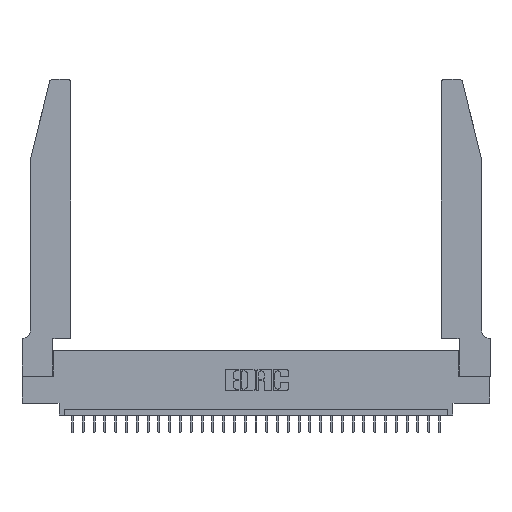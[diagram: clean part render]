
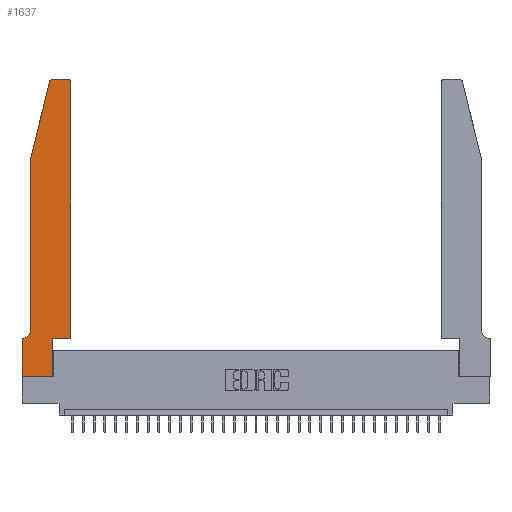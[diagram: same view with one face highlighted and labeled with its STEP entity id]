
A CAD part, top view. The second image highlights one B-rep face of the part: STEP entity #1637.
In plain terms, the highlighted planar face has unit normal (0, 0, 1).
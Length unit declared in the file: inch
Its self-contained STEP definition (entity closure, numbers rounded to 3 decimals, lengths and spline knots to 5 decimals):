
#861 = EDGE_CURVE ( 'NONE', #22324, #21856, #28466, .T. ) ;
#1229 = ORIENTED_EDGE ( 'NONE', *, *, #14745, .T. ) ;
#1288 = LINE ( 'NONE', #3930, #5575 ) ;
#1637 = ADVANCED_FACE ( 'NONE', ( #19854 ), #12151, .T. ) ;
#2127 = CARTESIAN_POINT ( 'NONE',  ( 0.0755, 2., 0.37 ) ) ;
#2329 = CARTESIAN_POINT ( 'NONE',  ( 0., 0.35, 0.37 ) ) ;
#2331 = CARTESIAN_POINT ( 'NONE',  ( 0.284, 2.72, 0.37 ) ) ;
#2631 = VERTEX_POINT ( 'NONE', #12043 ) ;
#2893 = VECTOR ( 'NONE', #9848, 39.37008 ) ;
#2916 = CARTESIAN_POINT ( 'NONE',  ( 0.2865, 0., 0.37 ) ) ;
#3930 = CARTESIAN_POINT ( 'NONE',  ( 0.0755, 0.35, 0.37 ) ) ;
#5282 = ORIENTED_EDGE ( 'NONE', *, *, #9246, .T. ) ;
#5521 = CARTESIAN_POINT ( 'NONE',  ( 0.0755, 2., 0.37 ) ) ;
#5575 = VECTOR ( 'NONE', #19083, 39.37008 ) ;
#5857 = EDGE_CURVE ( 'NONE', #2631, #22324, #8722, .T. ) ;
#5982 = DIRECTION ( 'NONE',  ( 0., 0., 1. ) ) ;
#6143 = CIRCLE ( 'NONE', #31142, 0.03 ) ;
#6165 = LINE ( 'NONE', #23189, #31897 ) ;
#6325 = VERTEX_POINT ( 'NONE', #20496 ) ;
#6509 = EDGE_CURVE ( 'NONE', #28198, #23085, #9923, .T. ) ;
#6625 = DIRECTION ( 'NONE',  ( 0., 0., -1. ) ) ;
#6813 = VERTEX_POINT ( 'NONE', #10339 ) ;
#6814 = EDGE_CURVE ( 'NONE', #6325, #8275, #25133, .T. ) ;
#7172 = CARTESIAN_POINT ( 'NONE',  ( 0.2865, 0.35, 0.37 ) ) ;
#7774 = AXIS2_PLACEMENT_3D ( 'NONE', #2329, #31929, #21804 ) ;
#8275 = VERTEX_POINT ( 'NONE', #2916 ) ;
#8722 = CIRCLE ( 'NONE', #31695, 0.03 ) ;
#9246 = EDGE_CURVE ( 'NONE', #29948, #19642, #29236, .T. ) ;
#9638 = LINE ( 'NONE', #16911, #32216 ) ;
#9848 = DIRECTION ( 'NONE',  ( 1., 0., 0. ) ) ;
#9882 = DIRECTION ( 'NONE',  ( 1., 0., 0. ) ) ;
#9923 = LINE ( 'NONE', #29613, #12692 ) ;
#9952 = DIRECTION ( 'NONE',  ( 1., 0., 0. ) ) ;
#9966 = CARTESIAN_POINT ( 'NONE',  ( 0., 0.35, 0.37 ) ) ;
#10187 = ORIENTED_EDGE ( 'NONE', *, *, #26667, .T. ) ;
#10339 = CARTESIAN_POINT ( 'NONE',  ( 0.0755, 0.42, 0.37 ) ) ;
#12043 = CARTESIAN_POINT ( 'NONE',  ( 0.4505, 2.72, 0.37 ) ) ;
#12145 = DIRECTION ( 'NONE',  ( 0., 1., 0. ) ) ;
#12151 = PLANE ( 'NONE',  #7774 ) ;
#12428 = ORIENTED_EDGE ( 'NONE', *, *, #6509, .T. ) ;
#12692 = VECTOR ( 'NONE', #9882, 39.37008 ) ;
#13392 = ORIENTED_EDGE ( 'NONE', *, *, #27468, .T. ) ;
#13490 = DIRECTION ( 'NONE',  ( 0., 1., 0. ) ) ;
#14745 = EDGE_CURVE ( 'NONE', #23166, #6325, #21315, .T. ) ;
#15244 = VECTOR ( 'NONE', #21880, 39.37008 ) ;
#16212 = CARTESIAN_POINT ( 'NONE',  ( 0.4205, 2.75, 0.37 ) ) ;
#16665 = CARTESIAN_POINT ( 'NONE',  ( 0.2605, 2.75, 0.37 ) ) ;
#16911 = CARTESIAN_POINT ( 'NONE',  ( 0.4505, 0.35, 0.37 ) ) ;
#18230 = VECTOR ( 'NONE', #24868, 39.37008 ) ;
#18362 = ORIENTED_EDGE ( 'NONE', *, *, #6814, .T. ) ;
#18542 = DIRECTION ( 'NONE',  ( 1., 0., 0. ) ) ;
#19083 = DIRECTION ( 'NONE',  ( -1., 0., 0. ) ) ;
#19445 = CARTESIAN_POINT ( 'NONE',  ( 0.4505, 0.35, 0.37 ) ) ;
#19642 = VERTEX_POINT ( 'NONE', #5521 ) ;
#19854 = FACE_OUTER_BOUND ( 'NONE', #26917, .T. ) ;
#20496 = CARTESIAN_POINT ( 'NONE',  ( 0., 0., 0.37 ) ) ;
#21029 = EDGE_CURVE ( 'NONE', #21856, #29948, #6143, .T. ) ;
#21315 = LINE ( 'NONE', #27130, #18230 ) ;
#21804 = DIRECTION ( 'NONE',  ( 1., 0., 0. ) ) ;
#21812 = VECTOR ( 'NONE', #29601, 39.37008 ) ;
#21856 = VERTEX_POINT ( 'NONE', #26995 ) ;
#21866 = VERTEX_POINT ( 'NONE', #29525 ) ;
#21880 = DIRECTION ( 'NONE',  ( -1., 0., 0. ) ) ;
#22016 = CARTESIAN_POINT ( 'NONE',  ( 0.0755, 2., 0.37 ) ) ;
#22324 = VERTEX_POINT ( 'NONE', #16212 ) ;
#23085 = VERTEX_POINT ( 'NONE', #19445 ) ;
#23166 = VERTEX_POINT ( 'NONE', #9966 ) ;
#23189 = CARTESIAN_POINT ( 'NONE',  ( 0.2865, 0.35, 0.37 ) ) ;
#23284 = ORIENTED_EDGE ( 'NONE', *, *, #5857, .T. ) ;
#23749 = CARTESIAN_POINT ( 'NONE',  ( 0., 0., 0.37 ) ) ;
#24390 = CARTESIAN_POINT ( 'NONE',  ( 0.0055, 0.42, 0.37 ) ) ;
#24817 = AXIS2_PLACEMENT_3D ( 'NONE', #24390, #6625, #31667 ) ;
#24868 = DIRECTION ( 'NONE',  ( 0., -1., 0. ) ) ;
#24899 = ORIENTED_EDGE ( 'NONE', *, *, #21029, .T. ) ;
#24960 = ORIENTED_EDGE ( 'NONE', *, *, #30134, .T. ) ;
#25133 = LINE ( 'NONE', #23749, #2893 ) ;
#25167 = ORIENTED_EDGE ( 'NONE', *, *, #27421, .T. ) ;
#25737 = CARTESIAN_POINT ( 'NONE',  ( 0.4205, 2.72, 0.37 ) ) ;
#26216 = LINE ( 'NONE', #22016, #27783 ) ;
#26667 = EDGE_CURVE ( 'NONE', #6813, #21866, #27846, .T. ) ;
#26680 = DIRECTION ( 'NONE',  ( 0., -1., 0. ) ) ;
#26917 = EDGE_LOOP ( 'NONE', ( #28869, #24899, #5282, #13392, #10187, #25167, #1229, #18362, #24960, #12428, #28415, #23284 ) ) ;
#26995 = CARTESIAN_POINT ( 'NONE',  ( 0.284, 2.75, 0.37 ) ) ;
#27130 = CARTESIAN_POINT ( 'NONE',  ( 0., 0., 0.37 ) ) ;
#27421 = EDGE_CURVE ( 'NONE', #21866, #23166, #1288, .T. ) ;
#27468 = EDGE_CURVE ( 'NONE', #19642, #6813, #26216, .T. ) ;
#27783 = VECTOR ( 'NONE', #26680, 39.37008 ) ;
#27846 = CIRCLE ( 'NONE', #24817, 0.07 ) ;
#28198 = VERTEX_POINT ( 'NONE', #7172 ) ;
#28415 = ORIENTED_EDGE ( 'NONE', *, *, #31087, .T. ) ;
#28466 = LINE ( 'NONE', #16665, #15244 ) ;
#28869 = ORIENTED_EDGE ( 'NONE', *, *, #861, .T. ) ;
#29236 = LINE ( 'NONE', #2127, #21812 ) ;
#29525 = CARTESIAN_POINT ( 'NONE',  ( 0.0055, 0.35, 0.37 ) ) ;
#29601 = DIRECTION ( 'NONE',  ( -0.239, -0.971, 0. ) ) ;
#29613 = CARTESIAN_POINT ( 'NONE',  ( 0.4505, 0.35, 0.37 ) ) ;
#29642 = CARTESIAN_POINT ( 'NONE',  ( 0.25487, 2.72718, 0.37 ) ) ;
#29948 = VERTEX_POINT ( 'NONE', #29642 ) ;
#30117 = DIRECTION ( 'NONE',  ( 0., 0., 1. ) ) ;
#30134 = EDGE_CURVE ( 'NONE', #8275, #28198, #6165, .T. ) ;
#31087 = EDGE_CURVE ( 'NONE', #23085, #2631, #9638, .T. ) ;
#31142 = AXIS2_PLACEMENT_3D ( 'NONE', #2331, #30117, #9952 ) ;
#31667 = DIRECTION ( 'NONE',  ( -1., 0., 0. ) ) ;
#31695 = AXIS2_PLACEMENT_3D ( 'NONE', #25737, #5982, #18542 ) ;
#31897 = VECTOR ( 'NONE', #13490, 39.37008 ) ;
#31929 = DIRECTION ( 'NONE',  ( 0., 0., 1. ) ) ;
#32216 = VECTOR ( 'NONE', #12145, 39.37008 ) ;
